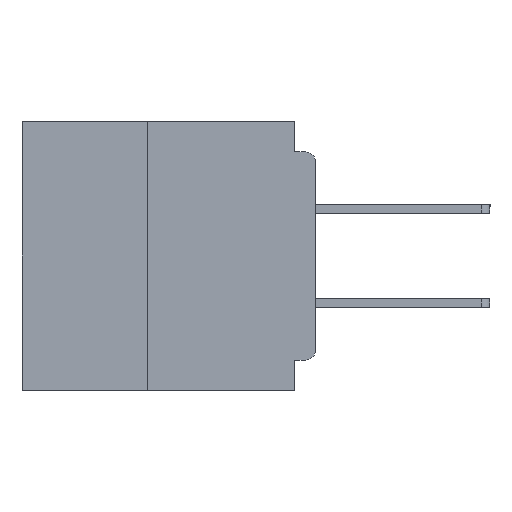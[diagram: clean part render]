
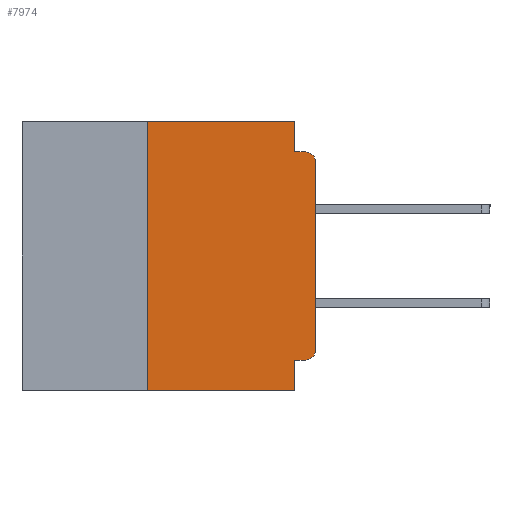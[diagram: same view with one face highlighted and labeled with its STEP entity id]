
A CAD part, left-side view. The second image highlights one B-rep face of the part: STEP entity #7974.
In plain terms, the highlighted planar face has unit normal (-1, 0, 0).
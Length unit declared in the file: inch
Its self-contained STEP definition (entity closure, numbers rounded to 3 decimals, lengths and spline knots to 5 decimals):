
#40 = EDGE_CURVE ( 'NONE', #12483, #7719, #9003, .T. ) ;
#90 = EDGE_CURVE ( 'NONE', #33412, #11714, #14574, .T. ) ;
#121 = ORIENTED_EDGE ( 'NONE', *, *, #27964, .F. ) ;
#317 = AXIS2_PLACEMENT_3D ( 'NONE', #2800, #26507, #27740 ) ;
#358 = LINE ( 'NONE', #17624, #28939 ) ;
#521 = VECTOR ( 'NONE', #18882, 39.37008 ) ;
#866 = DIRECTION ( 'NONE',  ( 0., 0., -1. ) ) ;
#1594 = VECTOR ( 'NONE', #9826, 39.37008 ) ;
#1670 = DIRECTION ( 'NONE',  ( 0., 0., -1. ) ) ;
#1901 = ORIENTED_EDGE ( 'NONE', *, *, #5646, .F. ) ;
#1963 = DIRECTION ( 'NONE',  ( 0., -1., 0. ) ) ;
#2393 = CARTESIAN_POINT ( 'NONE',  ( 0., 0., -0.355 ) ) ;
#2800 = CARTESIAN_POINT ( 'NONE',  ( 0., 0.015, -0.06 ) ) ;
#3218 = DIRECTION ( 'NONE',  ( 0., -1., 0. ) ) ;
#3353 = CARTESIAN_POINT ( 'NONE',  ( 0., 0.031, -0.045 ) ) ;
#4113 = CARTESIAN_POINT ( 'NONE',  ( 0., 0.031, -0.4 ) ) ;
#4532 = VECTOR ( 'NONE', #6904, 39.37008 ) ;
#5646 = EDGE_CURVE ( 'NONE', #32601, #17262, #358, .T. ) ;
#6904 = DIRECTION ( 'NONE',  ( 0., 0., -1. ) ) ;
#7141 = CARTESIAN_POINT ( 'NONE',  ( 0., 0.031, -0.4 ) ) ;
#7542 = CARTESIAN_POINT ( 'NONE',  ( 0., 0., -0.34 ) ) ;
#7561 = CARTESIAN_POINT ( 'NONE',  ( 0., 0.015, -0.355 ) ) ;
#7719 = VERTEX_POINT ( 'NONE', #24647 ) ;
#7974 = ADVANCED_FACE ( 'NONE', ( #13169 ), #25733, .F. ) ;
#8247 = VERTEX_POINT ( 'NONE', #7542 ) ;
#8629 = CARTESIAN_POINT ( 'NONE',  ( 0., 0., -0.06 ) ) ;
#9003 = LINE ( 'NONE', #10759, #1594 ) ;
#9642 = VECTOR ( 'NONE', #3218, 39.37008 ) ;
#9826 = DIRECTION ( 'NONE',  ( 0., 0., 1. ) ) ;
#10469 = LINE ( 'NONE', #15780, #24381 ) ;
#10576 = LINE ( 'NONE', #2393, #11439 ) ;
#10759 = CARTESIAN_POINT ( 'NONE',  ( 0., 0.25, -0.4 ) ) ;
#11439 = VECTOR ( 'NONE', #32886, 39.37008 ) ;
#11714 = VERTEX_POINT ( 'NONE', #16381 ) ;
#11867 = AXIS2_PLACEMENT_3D ( 'NONE', #31274, #17520, #866 ) ;
#12159 = VERTEX_POINT ( 'NONE', #7141 ) ;
#12483 = VERTEX_POINT ( 'NONE', #27163 ) ;
#12751 = LINE ( 'NONE', #4113, #4532 ) ;
#12893 = AXIS2_PLACEMENT_3D ( 'NONE', #34771, #18298, #1670 ) ;
#13070 = EDGE_LOOP ( 'NONE', ( #26187, #21419, #121, #1901, #16656, #25761, #33053, #19284, #34757, #28324 ) ) ;
#13169 = FACE_OUTER_BOUND ( 'NONE', #13070, .T. ) ;
#14112 = CARTESIAN_POINT ( 'NONE',  ( 0., 0.031, 0. ) ) ;
#14574 = CIRCLE ( 'NONE', #317, 0.015 ) ;
#14622 = VECTOR ( 'NONE', #35215, 39.37008 ) ;
#14985 = EDGE_CURVE ( 'NONE', #16179, #25830, #10576, .T. ) ;
#15518 = LINE ( 'NONE', #15980, #14622 ) ;
#15780 = CARTESIAN_POINT ( 'NONE',  ( 0., 0., -0.045 ) ) ;
#15980 = CARTESIAN_POINT ( 'NONE',  ( 0., 0., 0. ) ) ;
#16179 = VERTEX_POINT ( 'NONE', #7561 ) ;
#16381 = CARTESIAN_POINT ( 'NONE',  ( 0., 0.015, -0.045 ) ) ;
#16656 = ORIENTED_EDGE ( 'NONE', *, *, #27395, .F. ) ;
#17068 = CARTESIAN_POINT ( 'NONE',  ( 0., 0.437, -0.4 ) ) ;
#17262 = VERTEX_POINT ( 'NONE', #3353 ) ;
#17434 = DIRECTION ( 'NONE',  ( 0., 0., -1. ) ) ;
#17520 = DIRECTION ( 'NONE',  ( 1., 0., 0. ) ) ;
#17624 = CARTESIAN_POINT ( 'NONE',  ( 0., 0.031, 0. ) ) ;
#18298 = DIRECTION ( 'NONE',  ( -1., 0., 0. ) ) ;
#18433 = CIRCLE ( 'NONE', #12893, 0.015 ) ;
#18882 = DIRECTION ( 'NONE',  ( 0., -1., 0. ) ) ;
#19284 = ORIENTED_EDGE ( 'NONE', *, *, #32322, .F. ) ;
#19915 = EDGE_CURVE ( 'NONE', #8247, #33412, #15518, .T. ) ;
#21419 = ORIENTED_EDGE ( 'NONE', *, *, #90, .T. ) ;
#24381 = VECTOR ( 'NONE', #1963, 39.37008 ) ;
#24647 = CARTESIAN_POINT ( 'NONE',  ( 0., 0.25, 0. ) ) ;
#25733 = PLANE ( 'NONE',  #11867 ) ;
#25761 = ORIENTED_EDGE ( 'NONE', *, *, #40, .F. ) ;
#25830 = VERTEX_POINT ( 'NONE', #27361 ) ;
#26187 = ORIENTED_EDGE ( 'NONE', *, *, #19915, .T. ) ;
#26507 = DIRECTION ( 'NONE',  ( -1., 0., 0. ) ) ;
#27163 = CARTESIAN_POINT ( 'NONE',  ( 0., 0.25, -0.4 ) ) ;
#27361 = CARTESIAN_POINT ( 'NONE',  ( 0., 0.031, -0.355 ) ) ;
#27395 = EDGE_CURVE ( 'NONE', #7719, #32601, #30866, .T. ) ;
#27740 = DIRECTION ( 'NONE',  ( 0., 0., -1. ) ) ;
#27964 = EDGE_CURVE ( 'NONE', #17262, #11714, #10469, .T. ) ;
#28324 = ORIENTED_EDGE ( 'NONE', *, *, #32369, .T. ) ;
#28939 = VECTOR ( 'NONE', #17434, 39.37008 ) ;
#29957 = CARTESIAN_POINT ( 'NONE',  ( 0., 0.437, 0. ) ) ;
#30866 = LINE ( 'NONE', #29957, #521 ) ;
#31274 = CARTESIAN_POINT ( 'NONE',  ( 0., 0.437, 0. ) ) ;
#31726 = LINE ( 'NONE', #17068, #9642 ) ;
#32322 = EDGE_CURVE ( 'NONE', #25830, #12159, #12751, .T. ) ;
#32369 = EDGE_CURVE ( 'NONE', #16179, #8247, #18433, .T. ) ;
#32601 = VERTEX_POINT ( 'NONE', #14112 ) ;
#32886 = DIRECTION ( 'NONE',  ( 0., 1., 0. ) ) ;
#33053 = ORIENTED_EDGE ( 'NONE', *, *, #34119, .T. ) ;
#33412 = VERTEX_POINT ( 'NONE', #8629 ) ;
#34119 = EDGE_CURVE ( 'NONE', #12483, #12159, #31726, .T. ) ;
#34757 = ORIENTED_EDGE ( 'NONE', *, *, #14985, .F. ) ;
#34771 = CARTESIAN_POINT ( 'NONE',  ( 0., 0.015, -0.34 ) ) ;
#35215 = DIRECTION ( 'NONE',  ( 0., 0., 1. ) ) ;
